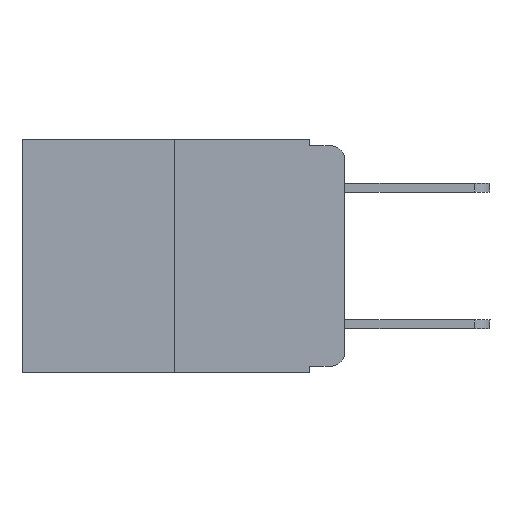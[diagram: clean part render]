
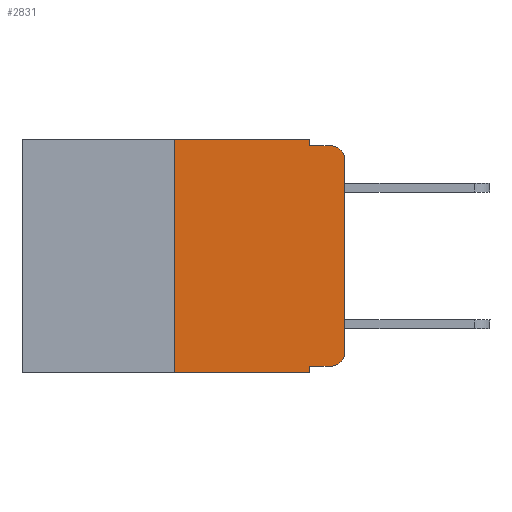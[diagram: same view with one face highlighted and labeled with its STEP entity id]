
A CAD part, left-side view. The second image highlights one B-rep face of the part: STEP entity #2831.
In plain terms, the highlighted planar face has unit normal (-1, 0, 0).
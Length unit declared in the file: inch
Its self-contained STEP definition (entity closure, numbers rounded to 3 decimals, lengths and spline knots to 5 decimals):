
#79 = VERTEX_POINT ( 'NONE', #14331 ) ;
#114 = ORIENTED_EDGE ( 'NONE', *, *, #3039, .F. ) ;
#183 = DIRECTION ( 'NONE',  ( 0., 0., -1. ) ) ;
#217 = LINE ( 'NONE', #10481, #12472 ) ;
#684 = EDGE_CURVE ( 'NONE', #7153, #1856, #4814, .T. ) ;
#766 = ORIENTED_EDGE ( 'NONE', *, *, #14947, .F. ) ;
#783 = VERTEX_POINT ( 'NONE', #2356 ) ;
#981 = DIRECTION ( 'NONE',  ( 0., -1., 0. ) ) ;
#1003 = CARTESIAN_POINT ( 'NONE',  ( 0., 0.25, 0. ) ) ;
#1640 = EDGE_CURVE ( 'NONE', #783, #14842, #13738, .T. ) ;
#1794 = EDGE_CURVE ( 'NONE', #11000, #11134, #217, .T. ) ;
#1856 = VERTEX_POINT ( 'NONE', #11842 ) ;
#2085 = DIRECTION ( 'NONE',  ( 0., 0., -1. ) ) ;
#2356 = CARTESIAN_POINT ( 'NONE',  ( 0., 0.25, -0.343 ) ) ;
#2831 = ADVANCED_FACE ( 'NONE', ( #16057 ), #13451, .F. ) ;
#3039 = EDGE_CURVE ( 'NONE', #14842, #7153, #3055, .T. ) ;
#3055 = LINE ( 'NONE', #8173, #16033 ) ;
#3453 = ORIENTED_EDGE ( 'NONE', *, *, #1640, .F. ) ;
#3729 = EDGE_CURVE ( 'NONE', #7674, #5491, #6112, .T. ) ;
#3808 = ORIENTED_EDGE ( 'NONE', *, *, #10299, .F. ) ;
#4017 = DIRECTION ( 'NONE',  ( 0., -1., 0. ) ) ;
#4172 = CARTESIAN_POINT ( 'NONE',  ( 0., 0.02, -0.03 ) ) ;
#4321 = EDGE_LOOP ( 'NONE', ( #4780, #16013, #3808, #13339, #114, #3453, #5754, #766, #12308, #4743 ) ) ;
#4359 = CARTESIAN_POINT ( 'NONE',  ( 0., 0.473, 0. ) ) ;
#4713 = VECTOR ( 'NONE', #4017, 39.37008 ) ;
#4743 = ORIENTED_EDGE ( 'NONE', *, *, #6610, .T. ) ;
#4780 = ORIENTED_EDGE ( 'NONE', *, *, #1794, .T. ) ;
#4814 = LINE ( 'NONE', #7214, #6225 ) ;
#5051 = DIRECTION ( 'NONE',  ( -1., 0., 0. ) ) ;
#5098 = CARTESIAN_POINT ( 'NONE',  ( 0., 0.051, -0.343 ) ) ;
#5491 = VERTEX_POINT ( 'NONE', #13781 ) ;
#5505 = DIRECTION ( 'NONE',  ( 0., -1., 0. ) ) ;
#5658 = VERTEX_POINT ( 'NONE', #5098 ) ;
#5743 = DIRECTION ( 'NONE',  ( 0., 0., -1. ) ) ;
#5754 = ORIENTED_EDGE ( 'NONE', *, *, #12963, .T. ) ;
#5972 = LINE ( 'NONE', #14830, #8055 ) ;
#6112 = LINE ( 'NONE', #7189, #9836 ) ;
#6225 = VECTOR ( 'NONE', #5743, 39.37008 ) ;
#6335 = CARTESIAN_POINT ( 'NONE',  ( 0., 0.473, -0.343 ) ) ;
#6610 = EDGE_CURVE ( 'NONE', #5491, #11000, #13997, .T. ) ;
#7153 = VERTEX_POINT ( 'NONE', #8027 ) ;
#7189 = CARTESIAN_POINT ( 'NONE',  ( 0., 0.051, -0.333 ) ) ;
#7214 = CARTESIAN_POINT ( 'NONE',  ( 0., 0.051, 0. ) ) ;
#7487 = CARTESIAN_POINT ( 'NONE',  ( 0., 0., -0.313 ) ) ;
#7601 = LINE ( 'NONE', #6335, #11010 ) ;
#7674 = VERTEX_POINT ( 'NONE', #15796 ) ;
#7754 = EDGE_CURVE ( 'NONE', #11134, #79, #9685, .T. ) ;
#7796 = CARTESIAN_POINT ( 'NONE',  ( 0., 0.02, -0.313 ) ) ;
#8027 = CARTESIAN_POINT ( 'NONE',  ( 0., 0.051, 0. ) ) ;
#8055 = VECTOR ( 'NONE', #2085, 39.37008 ) ;
#8173 = CARTESIAN_POINT ( 'NONE',  ( 0., 0.473, 0. ) ) ;
#8685 = VECTOR ( 'NONE', #15090, 39.37008 ) ;
#8858 = AXIS2_PLACEMENT_3D ( 'NONE', #7796, #5051, #12968 ) ;
#9685 = CIRCLE ( 'NONE', #14581, 0.02 ) ;
#9836 = VECTOR ( 'NONE', #981, 39.37008 ) ;
#10111 = CARTESIAN_POINT ( 'NONE',  ( 0., 0., -0.03 ) ) ;
#10299 = EDGE_CURVE ( 'NONE', #1856, #79, #12868, .T. ) ;
#10481 = CARTESIAN_POINT ( 'NONE',  ( 0., 0., 0. ) ) ;
#10684 = CARTESIAN_POINT ( 'NONE',  ( 0., 0.25, 0. ) ) ;
#10824 = DIRECTION ( 'NONE',  ( 1., 0., 0. ) ) ;
#11000 = VERTEX_POINT ( 'NONE', #7487 ) ;
#11010 = VECTOR ( 'NONE', #11399, 39.37008 ) ;
#11134 = VERTEX_POINT ( 'NONE', #10111 ) ;
#11161 = AXIS2_PLACEMENT_3D ( 'NONE', #4359, #10824, #12082 ) ;
#11399 = DIRECTION ( 'NONE',  ( 0., -1., 0. ) ) ;
#11594 = CARTESIAN_POINT ( 'NONE',  ( 0., 0.051, -0.01 ) ) ;
#11842 = CARTESIAN_POINT ( 'NONE',  ( 0., 0.051, -0.01 ) ) ;
#12082 = DIRECTION ( 'NONE',  ( 0., 0., -1. ) ) ;
#12308 = ORIENTED_EDGE ( 'NONE', *, *, #3729, .T. ) ;
#12472 = VECTOR ( 'NONE', #15664, 39.37008 ) ;
#12868 = LINE ( 'NONE', #11594, #4713 ) ;
#12963 = EDGE_CURVE ( 'NONE', #783, #5658, #7601, .T. ) ;
#12968 = DIRECTION ( 'NONE',  ( 0., 0., -1. ) ) ;
#13339 = ORIENTED_EDGE ( 'NONE', *, *, #684, .F. ) ;
#13451 = PLANE ( 'NONE',  #11161 ) ;
#13738 = LINE ( 'NONE', #1003, #8685 ) ;
#13781 = CARTESIAN_POINT ( 'NONE',  ( 0., 0.02, -0.333 ) ) ;
#13997 = CIRCLE ( 'NONE', #8858, 0.02 ) ;
#14331 = CARTESIAN_POINT ( 'NONE',  ( 0., 0.02, -0.01 ) ) ;
#14447 = DIRECTION ( 'NONE',  ( -1., 0., 0. ) ) ;
#14581 = AXIS2_PLACEMENT_3D ( 'NONE', #4172, #14447, #183 ) ;
#14830 = CARTESIAN_POINT ( 'NONE',  ( 0., 0.051, 0. ) ) ;
#14842 = VERTEX_POINT ( 'NONE', #10684 ) ;
#14947 = EDGE_CURVE ( 'NONE', #7674, #5658, #5972, .T. ) ;
#15090 = DIRECTION ( 'NONE',  ( 0., 0., 1. ) ) ;
#15664 = DIRECTION ( 'NONE',  ( 0., 0., 1. ) ) ;
#15796 = CARTESIAN_POINT ( 'NONE',  ( 0., 0.051, -0.333 ) ) ;
#16013 = ORIENTED_EDGE ( 'NONE', *, *, #7754, .T. ) ;
#16033 = VECTOR ( 'NONE', #5505, 39.37008 ) ;
#16057 = FACE_OUTER_BOUND ( 'NONE', #4321, .T. ) ;
